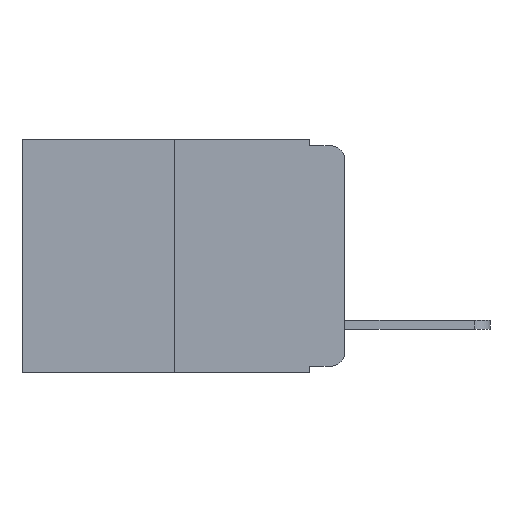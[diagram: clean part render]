
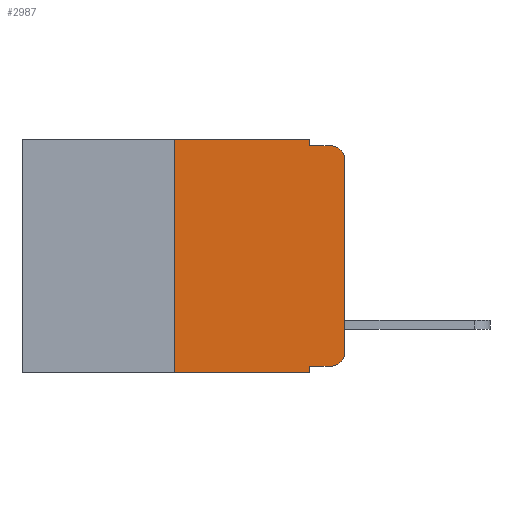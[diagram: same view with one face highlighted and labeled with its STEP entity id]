
A CAD part, left-side view. The second image highlights one B-rep face of the part: STEP entity #2987.
In plain terms, the highlighted planar face has unit normal (-1, 0, 0).
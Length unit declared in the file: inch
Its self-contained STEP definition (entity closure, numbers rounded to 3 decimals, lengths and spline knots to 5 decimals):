
#242 = CIRCLE ( 'NONE', #10861, 0.02 ) ;
#688 = VECTOR ( 'NONE', #19980, 39.37008 ) ;
#756 = CARTESIAN_POINT ( 'NONE',  ( 0., 0.02, -0.03 ) ) ;
#768 = VERTEX_POINT ( 'NONE', #9882 ) ;
#832 = DIRECTION ( 'NONE',  ( -1., 0., 0. ) ) ;
#1214 = LINE ( 'NONE', #7781, #6766 ) ;
#1500 = ORIENTED_EDGE ( 'NONE', *, *, #11390, .F. ) ;
#2108 = ORIENTED_EDGE ( 'NONE', *, *, #12877, .F. ) ;
#2394 = ORIENTED_EDGE ( 'NONE', *, *, #23947, .F. ) ;
#2758 = ORIENTED_EDGE ( 'NONE', *, *, #9174, .F. ) ;
#2868 = VECTOR ( 'NONE', #22119, 39.37008 ) ;
#2906 = DIRECTION ( 'NONE',  ( 0., 0., -1. ) ) ;
#2987 = ADVANCED_FACE ( 'NONE', ( #17062 ), #7050, .F. ) ;
#4038 = ORIENTED_EDGE ( 'NONE', *, *, #10233, .T. ) ;
#4080 = CARTESIAN_POINT ( 'NONE',  ( 0., 0.02, -0.333 ) ) ;
#4975 = CARTESIAN_POINT ( 'NONE',  ( 0., 0.473, -0.343 ) ) ;
#5300 = DIRECTION ( 'NONE',  ( 0., -1., 0. ) ) ;
#5321 = CARTESIAN_POINT ( 'NONE',  ( 0., 0.02, -0.01 ) ) ;
#5506 = AXIS2_PLACEMENT_3D ( 'NONE', #756, #832, #17606 ) ;
#5744 = ORIENTED_EDGE ( 'NONE', *, *, #13129, .T. ) ;
#5823 = DIRECTION ( 'NONE',  ( 0., 0., 1. ) ) ;
#5932 = EDGE_CURVE ( 'NONE', #8438, #13964, #242, .T. ) ;
#5966 = EDGE_CURVE ( 'NONE', #768, #9080, #14288, .T. ) ;
#6766 = VECTOR ( 'NONE', #5823, 39.37008 ) ;
#6876 = CARTESIAN_POINT ( 'NONE',  ( 0., 0.051, 0. ) ) ;
#7050 = PLANE ( 'NONE',  #14765 ) ;
#7066 = CARTESIAN_POINT ( 'NONE',  ( 0., 0.051, 0. ) ) ;
#7422 = ORIENTED_EDGE ( 'NONE', *, *, #21845, .T. ) ;
#7781 = CARTESIAN_POINT ( 'NONE',  ( 0., 0., 0. ) ) ;
#7872 = EDGE_LOOP ( 'NONE', ( #7422, #4038, #1500, #2758, #2108, #2394, #5744, #10002, #22227, #17344 ) ) ;
#8002 = VECTOR ( 'NONE', #24020, 39.37008 ) ;
#8252 = DIRECTION ( 'NONE',  ( 0., -1., 0. ) ) ;
#8438 = VERTEX_POINT ( 'NONE', #4080 ) ;
#9080 = VERTEX_POINT ( 'NONE', #9609 ) ;
#9086 = LINE ( 'NONE', #4975, #20512 ) ;
#9174 = EDGE_CURVE ( 'NONE', #21295, #22938, #17099, .T. ) ;
#9204 = EDGE_CURVE ( 'NONE', #768, #8438, #19152, .T. ) ;
#9290 = VERTEX_POINT ( 'NONE', #21487 ) ;
#9609 = CARTESIAN_POINT ( 'NONE',  ( 0., 0.051, -0.343 ) ) ;
#9882 = CARTESIAN_POINT ( 'NONE',  ( 0., 0.051, -0.333 ) ) ;
#10002 = ORIENTED_EDGE ( 'NONE', *, *, #5966, .F. ) ;
#10233 = EDGE_CURVE ( 'NONE', #12337, #21678, #18806, .T. ) ;
#10555 = CARTESIAN_POINT ( 'NONE',  ( 0., 0.051, 0. ) ) ;
#10861 = AXIS2_PLACEMENT_3D ( 'NONE', #23516, #23677, #2906 ) ;
#11302 = CARTESIAN_POINT ( 'NONE',  ( 0., 0.051, -0.01 ) ) ;
#11390 = EDGE_CURVE ( 'NONE', #22938, #21678, #16817, .T. ) ;
#12326 = VECTOR ( 'NONE', #8252, 39.37008 ) ;
#12337 = VERTEX_POINT ( 'NONE', #19599 ) ;
#12877 = EDGE_CURVE ( 'NONE', #9290, #21295, #23166, .T. ) ;
#13129 = EDGE_CURVE ( 'NONE', #14445, #9080, #9086, .T. ) ;
#13964 = VERTEX_POINT ( 'NONE', #23370 ) ;
#14288 = LINE ( 'NONE', #10555, #15493 ) ;
#14334 = CARTESIAN_POINT ( 'NONE',  ( 0., 0.473, 0. ) ) ;
#14425 = VECTOR ( 'NONE', #16789, 39.37008 ) ;
#14445 = VERTEX_POINT ( 'NONE', #23181 ) ;
#14765 = AXIS2_PLACEMENT_3D ( 'NONE', #14334, #21922, #16398 ) ;
#15493 = VECTOR ( 'NONE', #20003, 39.37008 ) ;
#16398 = DIRECTION ( 'NONE',  ( 0., 0., -1. ) ) ;
#16635 = CARTESIAN_POINT ( 'NONE',  ( 0., 0.051, -0.333 ) ) ;
#16789 = DIRECTION ( 'NONE',  ( 0., -1., 0. ) ) ;
#16817 = LINE ( 'NONE', #20270, #8002 ) ;
#17062 = FACE_OUTER_BOUND ( 'NONE', #7872, .T. ) ;
#17099 = LINE ( 'NONE', #6876, #688 ) ;
#17344 = ORIENTED_EDGE ( 'NONE', *, *, #5932, .T. ) ;
#17528 = CARTESIAN_POINT ( 'NONE',  ( 0., 0.473, 0. ) ) ;
#17606 = DIRECTION ( 'NONE',  ( 0., 0., -1. ) ) ;
#18714 = LINE ( 'NONE', #20262, #2868 ) ;
#18806 = CIRCLE ( 'NONE', #5506, 0.02 ) ;
#19152 = LINE ( 'NONE', #16635, #14425 ) ;
#19599 = CARTESIAN_POINT ( 'NONE',  ( 0., 0., -0.03 ) ) ;
#19980 = DIRECTION ( 'NONE',  ( 0., 0., -1. ) ) ;
#20003 = DIRECTION ( 'NONE',  ( 0., 0., -1. ) ) ;
#20262 = CARTESIAN_POINT ( 'NONE',  ( 0., 0.25, 0. ) ) ;
#20270 = CARTESIAN_POINT ( 'NONE',  ( 0., 0.051, -0.01 ) ) ;
#20512 = VECTOR ( 'NONE', #5300, 39.37008 ) ;
#21295 = VERTEX_POINT ( 'NONE', #7066 ) ;
#21487 = CARTESIAN_POINT ( 'NONE',  ( 0., 0.25, 0. ) ) ;
#21678 = VERTEX_POINT ( 'NONE', #5321 ) ;
#21845 = EDGE_CURVE ( 'NONE', #13964, #12337, #1214, .T. ) ;
#21922 = DIRECTION ( 'NONE',  ( 1., 0., 0. ) ) ;
#22119 = DIRECTION ( 'NONE',  ( 0., 0., 1. ) ) ;
#22227 = ORIENTED_EDGE ( 'NONE', *, *, #9204, .T. ) ;
#22938 = VERTEX_POINT ( 'NONE', #11302 ) ;
#23166 = LINE ( 'NONE', #17528, #12326 ) ;
#23181 = CARTESIAN_POINT ( 'NONE',  ( 0., 0.25, -0.343 ) ) ;
#23370 = CARTESIAN_POINT ( 'NONE',  ( 0., 0., -0.313 ) ) ;
#23516 = CARTESIAN_POINT ( 'NONE',  ( 0., 0.02, -0.313 ) ) ;
#23677 = DIRECTION ( 'NONE',  ( -1., 0., 0. ) ) ;
#23947 = EDGE_CURVE ( 'NONE', #14445, #9290, #18714, .T. ) ;
#24020 = DIRECTION ( 'NONE',  ( 0., -1., 0. ) ) ;
